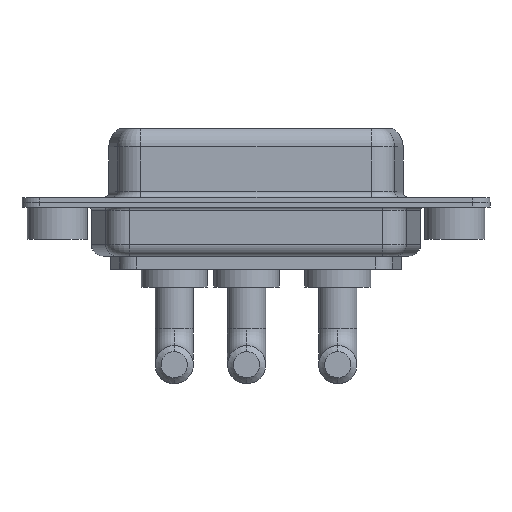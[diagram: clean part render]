
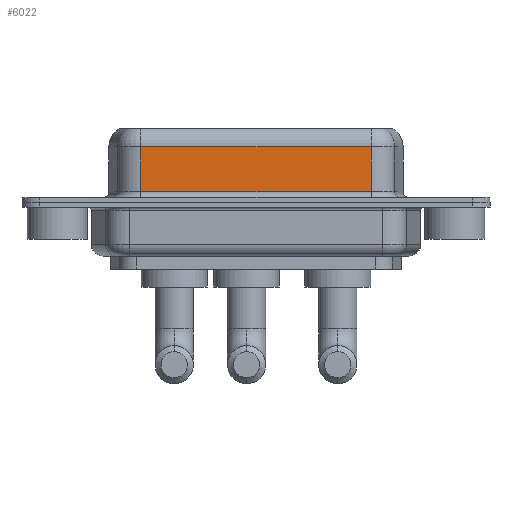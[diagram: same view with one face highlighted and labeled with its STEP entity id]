
A CAD part, front view. The second image highlights one B-rep face of the part: STEP entity #6022.
In plain terms, the highlighted planar face has unit normal (0, -1, 0).
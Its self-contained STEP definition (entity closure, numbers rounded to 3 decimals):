
#579 = EDGE_CURVE ( 'NONE', #10848, #8295, #10841, .T. ) ;
#1248 = VECTOR ( 'NONE', #3372, 1000. ) ;
#1670 = CARTESIAN_POINT ( 'NONE',  ( 26.287, -3.95, 6.4 ) ) ;
#2037 = CARTESIAN_POINT ( 'NONE',  ( 7.013, -3.95, 6.4 ) ) ;
#2046 = DIRECTION ( 'NONE',  ( 1., 0., 0. ) ) ;
#2505 = DIRECTION ( 'NONE',  ( -1., 0., 0. ) ) ;
#3372 = DIRECTION ( 'NONE',  ( 0., 0., -1. ) ) ;
#3384 = LINE ( 'NONE', #4300, #3406 ) ;
#3406 = VECTOR ( 'NONE', #2046, 1000. ) ;
#4300 = CARTESIAN_POINT ( 'NONE',  ( 26.287, -3.95, 0.9 ) ) ;
#4504 = CARTESIAN_POINT ( 'NONE',  ( 26.287, -3.95, 0.9 ) ) ;
#5159 = VECTOR ( 'NONE', #2505, 1000. ) ;
#5312 = CARTESIAN_POINT ( 'NONE',  ( 26.287, -3.95, 6.4 ) ) ;
#6022 = ADVANCED_FACE ( 'NONE', ( #7546 ), #11883, .F. ) ;
#6448 = VERTEX_POINT ( 'NONE', #4504 ) ;
#6782 = ORIENTED_EDGE ( 'NONE', *, *, #579, .T. ) ;
#6857 = VECTOR ( 'NONE', #10168, 1000. ) ;
#7306 = EDGE_CURVE ( 'NONE', #13145, #6448, #3384, .T. ) ;
#7546 = FACE_OUTER_BOUND ( 'NONE', #12124, .T. ) ;
#7780 = AXIS2_PLACEMENT_3D ( 'NONE', #5312, #11814, #12782 ) ;
#8196 = LINE ( 'NONE', #1670, #6857 ) ;
#8295 = VERTEX_POINT ( 'NONE', #11385 ) ;
#8944 = CARTESIAN_POINT ( 'NONE',  ( 26.287, -3.95, 4.65 ) ) ;
#9043 = EDGE_CURVE ( 'NONE', #8295, #13145, #12676, .T. ) ;
#9251 = CARTESIAN_POINT ( 'NONE',  ( 7.013, -3.95, 0.9 ) ) ;
#10168 = DIRECTION ( 'NONE',  ( 0., 0., -1. ) ) ;
#10352 = ORIENTED_EDGE ( 'NONE', *, *, #9043, .T. ) ;
#10841 = LINE ( 'NONE', #12102, #5159 ) ;
#10848 = VERTEX_POINT ( 'NONE', #8944 ) ;
#11270 = EDGE_CURVE ( 'NONE', #10848, #6448, #8196, .T. ) ;
#11340 = ORIENTED_EDGE ( 'NONE', *, *, #11270, .F. ) ;
#11385 = CARTESIAN_POINT ( 'NONE',  ( 7.013, -3.95, 4.65 ) ) ;
#11814 = DIRECTION ( 'NONE',  ( 0., 1., 0. ) ) ;
#11854 = ORIENTED_EDGE ( 'NONE', *, *, #7306, .T. ) ;
#11883 = PLANE ( 'NONE',  #7780 ) ;
#12102 = CARTESIAN_POINT ( 'NONE',  ( 26.287, -3.95, 4.65 ) ) ;
#12124 = EDGE_LOOP ( 'NONE', ( #11340, #6782, #10352, #11854 ) ) ;
#12676 = LINE ( 'NONE', #2037, #1248 ) ;
#12782 = DIRECTION ( 'NONE',  ( 0., 0., 1. ) ) ;
#13145 = VERTEX_POINT ( 'NONE', #9251 ) ;
